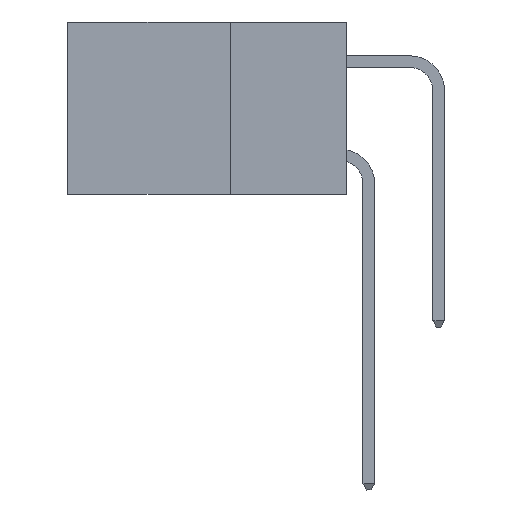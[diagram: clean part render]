
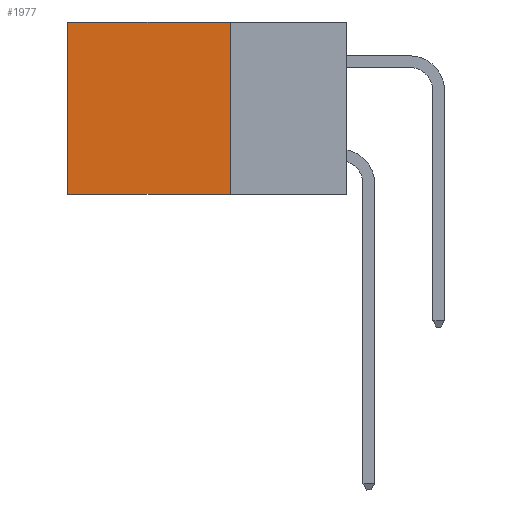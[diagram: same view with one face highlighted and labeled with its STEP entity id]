
A CAD part, left-side view. The second image highlights one B-rep face of the part: STEP entity #1977.
In plain terms, the highlighted planar face has unit normal (-1, 0, 0).
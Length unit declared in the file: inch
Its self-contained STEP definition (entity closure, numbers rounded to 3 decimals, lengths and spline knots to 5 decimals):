
#506 = EDGE_LOOP ( 'NONE', ( #11612, #4386, #7569, #12062 ) ) ;
#997 = FACE_OUTER_BOUND ( 'NONE', #506, .T. ) ;
#1438 = VERTEX_POINT ( 'NONE', #4231 ) ;
#1495 = PLANE ( 'NONE',  #12296 ) ;
#1977 = ADVANCED_FACE ( 'NONE', ( #997 ), #1495, .F. ) ;
#2259 = LINE ( 'NONE', #7471, #4299 ) ;
#2283 = DIRECTION ( 'NONE',  ( 0., 0., -1. ) ) ;
#4010 = LINE ( 'NONE', #5845, #9703 ) ;
#4231 = CARTESIAN_POINT ( 'NONE',  ( 0.2875, 0.25, -0.37 ) ) ;
#4299 = VECTOR ( 'NONE', #8533, 39.37008 ) ;
#4386 = ORIENTED_EDGE ( 'NONE', *, *, #8294, .F. ) ;
#5146 = DIRECTION ( 'NONE',  ( 0., 0., -1. ) ) ;
#5845 = CARTESIAN_POINT ( 'NONE',  ( 0.2875, 0.25, 0. ) ) ;
#6094 = VERTEX_POINT ( 'NONE', #14746 ) ;
#6560 = DIRECTION ( 'NONE',  ( 0., 0., -1. ) ) ;
#6772 = EDGE_CURVE ( 'NONE', #9574, #6094, #2259, .T. ) ;
#7471 = CARTESIAN_POINT ( 'NONE',  ( 0.2875, 0.25, 0. ) ) ;
#7569 = ORIENTED_EDGE ( 'NONE', *, *, #18571, .F. ) ;
#8294 = EDGE_CURVE ( 'NONE', #1438, #16013, #16463, .T. ) ;
#8348 = EDGE_CURVE ( 'NONE', #6094, #16013, #8614, .T. ) ;
#8533 = DIRECTION ( 'NONE',  ( 0., 1., 0. ) ) ;
#8614 = LINE ( 'NONE', #11034, #16913 ) ;
#9574 = VERTEX_POINT ( 'NONE', #18466 ) ;
#9703 = VECTOR ( 'NONE', #2283, 39.37008 ) ;
#11034 = CARTESIAN_POINT ( 'NONE',  ( 0.2875, 0.6, 0. ) ) ;
#11612 = ORIENTED_EDGE ( 'NONE', *, *, #8348, .T. ) ;
#11767 = CARTESIAN_POINT ( 'NONE',  ( 0.2875, 0.25, 0. ) ) ;
#12062 = ORIENTED_EDGE ( 'NONE', *, *, #6772, .T. ) ;
#12151 = CARTESIAN_POINT ( 'NONE',  ( 0.2875, 0.25, -0.37 ) ) ;
#12296 = AXIS2_PLACEMENT_3D ( 'NONE', #11767, #15254, #5146 ) ;
#12525 = VECTOR ( 'NONE', #13848, 39.37008 ) ;
#13848 = DIRECTION ( 'NONE',  ( 0., 1., 0. ) ) ;
#14121 = CARTESIAN_POINT ( 'NONE',  ( 0.2875, 0.6, -0.37 ) ) ;
#14746 = CARTESIAN_POINT ( 'NONE',  ( 0.2875, 0.6, 0. ) ) ;
#15254 = DIRECTION ( 'NONE',  ( 1., 0., 0. ) ) ;
#16013 = VERTEX_POINT ( 'NONE', #14121 ) ;
#16463 = LINE ( 'NONE', #12151, #12525 ) ;
#16913 = VECTOR ( 'NONE', #6560, 39.37008 ) ;
#18466 = CARTESIAN_POINT ( 'NONE',  ( 0.2875, 0.25, 0. ) ) ;
#18571 = EDGE_CURVE ( 'NONE', #9574, #1438, #4010, .T. ) ;
